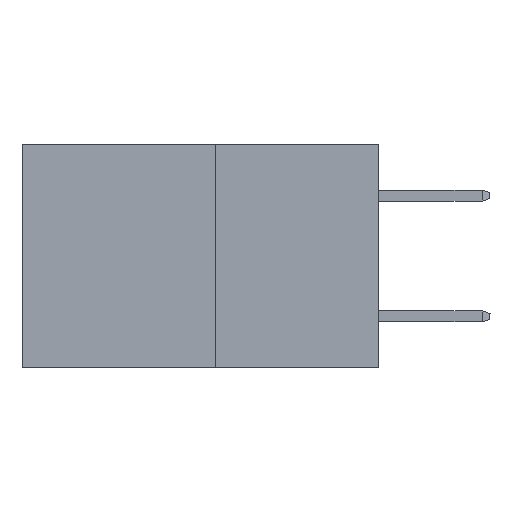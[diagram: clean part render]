
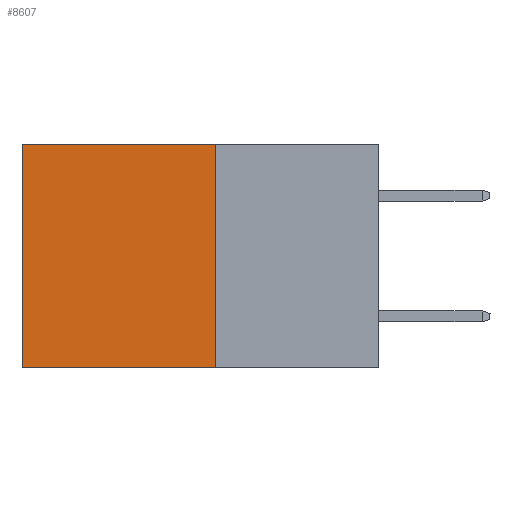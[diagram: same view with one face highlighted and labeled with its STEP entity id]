
A CAD part, left-side view. The second image highlights one B-rep face of the part: STEP entity #8607.
In plain terms, the highlighted planar face has unit normal (-1, 0, 0).
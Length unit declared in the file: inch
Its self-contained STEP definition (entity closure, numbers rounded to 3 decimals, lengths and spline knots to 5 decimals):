
#404 = CARTESIAN_POINT ( 'NONE',  ( 0.277, 0.27, 0. ) ) ;
#644 = ORIENTED_EDGE ( 'NONE', *, *, #15311, .T. ) ;
#1535 = DIRECTION ( 'NONE',  ( 0., 0., -1. ) ) ;
#2394 = CARTESIAN_POINT ( 'NONE',  ( 0.277, 0.27, -0.37 ) ) ;
#5057 = CARTESIAN_POINT ( 'NONE',  ( 0.277, 0.27, 0. ) ) ;
#5339 = LINE ( 'NONE', #15546, #23505 ) ;
#5438 = VECTOR ( 'NONE', #28748, 39.37008 ) ;
#6087 = CARTESIAN_POINT ( 'NONE',  ( 0.277, 0.59, 0. ) ) ;
#6194 = LINE ( 'NONE', #5057, #5438 ) ;
#6266 = EDGE_CURVE ( 'NONE', #29903, #6804, #19864, .T. ) ;
#6804 = VERTEX_POINT ( 'NONE', #19028 ) ;
#8142 = EDGE_CURVE ( 'NONE', #22172, #29903, #10913, .T. ) ;
#8274 = ORIENTED_EDGE ( 'NONE', *, *, #8142, .F. ) ;
#8607 = ADVANCED_FACE ( 'NONE', ( #11620 ), #13474, .F. ) ;
#10049 = CARTESIAN_POINT ( 'NONE',  ( 0.277, 0.27, -0.37 ) ) ;
#10913 = LINE ( 'NONE', #2394, #17214 ) ;
#11620 = FACE_OUTER_BOUND ( 'NONE', #15624, .T. ) ;
#13474 = PLANE ( 'NONE',  #22174 ) ;
#13586 = VECTOR ( 'NONE', #24294, 39.37008 ) ;
#15311 = EDGE_CURVE ( 'NONE', #22172, #26627, #6194, .T. ) ;
#15546 = CARTESIAN_POINT ( 'NONE',  ( 0.277, 0.59, -0.37 ) ) ;
#15624 = EDGE_LOOP ( 'NONE', ( #25395, #17246, #8274, #644 ) ) ;
#15706 = CARTESIAN_POINT ( 'NONE',  ( 0.277, 0.27, -0.37 ) ) ;
#15849 = DIRECTION ( 'NONE',  ( 1., 0., 0. ) ) ;
#17214 = VECTOR ( 'NONE', #26055, 39.37008 ) ;
#17246 = ORIENTED_EDGE ( 'NONE', *, *, #6266, .F. ) ;
#19028 = CARTESIAN_POINT ( 'NONE',  ( 0.277, 0.59, -0.37 ) ) ;
#19864 = LINE ( 'NONE', #10049, #13586 ) ;
#20239 = EDGE_CURVE ( 'NONE', #26627, #6804, #5339, .T. ) ;
#22172 = VERTEX_POINT ( 'NONE', #404 ) ;
#22174 = AXIS2_PLACEMENT_3D ( 'NONE', #29949, #15849, #1535 ) ;
#23505 = VECTOR ( 'NONE', #24919, 39.37008 ) ;
#24294 = DIRECTION ( 'NONE',  ( 0., 1., 0. ) ) ;
#24919 = DIRECTION ( 'NONE',  ( 0., 0., -1. ) ) ;
#25395 = ORIENTED_EDGE ( 'NONE', *, *, #20239, .T. ) ;
#26055 = DIRECTION ( 'NONE',  ( 0., 0., -1. ) ) ;
#26627 = VERTEX_POINT ( 'NONE', #6087 ) ;
#28748 = DIRECTION ( 'NONE',  ( 0., 1., 0. ) ) ;
#29903 = VERTEX_POINT ( 'NONE', #15706 ) ;
#29949 = CARTESIAN_POINT ( 'NONE',  ( 0.277, 0.27, -0.37 ) ) ;
